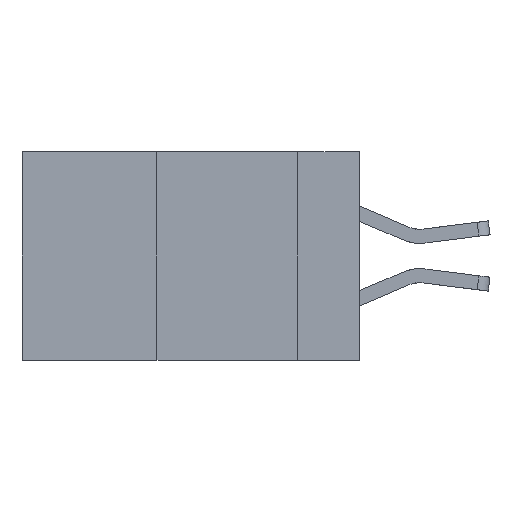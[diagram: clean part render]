
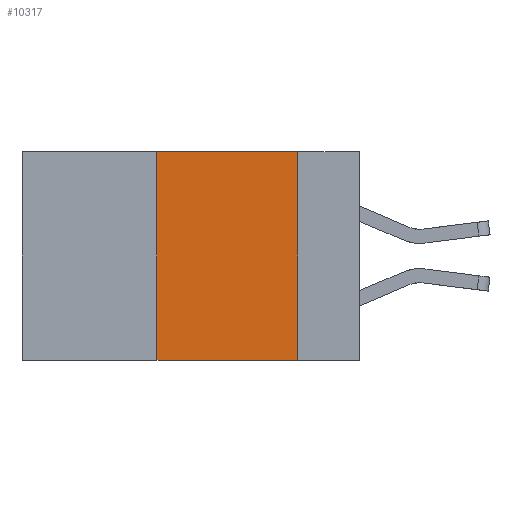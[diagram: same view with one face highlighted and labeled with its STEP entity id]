
A CAD part, left-side view. The second image highlights one B-rep face of the part: STEP entity #10317.
In plain terms, the highlighted planar face has unit normal (-1, 0, 0).
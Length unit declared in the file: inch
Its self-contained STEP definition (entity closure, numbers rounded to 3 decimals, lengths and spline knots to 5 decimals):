
#854 = VECTOR ( 'NONE', #16320, 39.37008 ) ;
#1906 = VECTOR ( 'NONE', #15394, 39.37008 ) ;
#2487 = LINE ( 'NONE', #2749, #8950 ) ;
#2667 = ORIENTED_EDGE ( 'NONE', *, *, #12969, .F. ) ;
#2749 = CARTESIAN_POINT ( 'NONE',  ( 0., 0.6, -0.37 ) ) ;
#3120 = DIRECTION ( 'NONE',  ( 0., 0., -1. ) ) ;
#3386 = VERTEX_POINT ( 'NONE', #4968 ) ;
#3790 = VERTEX_POINT ( 'NONE', #15753 ) ;
#4628 = EDGE_CURVE ( 'NONE', #3386, #15463, #11098, .T. ) ;
#4667 = ORIENTED_EDGE ( 'NONE', *, *, #4628, .F. ) ;
#4968 = CARTESIAN_POINT ( 'NONE',  ( 0., 0.11, 0. ) ) ;
#5385 = DIRECTION ( 'NONE',  ( 0., -1., 0. ) ) ;
#5990 = FACE_OUTER_BOUND ( 'NONE', #14815, .T. ) ;
#7098 = DIRECTION ( 'NONE',  ( 0., -1., 0. ) ) ;
#7210 = LINE ( 'NONE', #14606, #13504 ) ;
#8582 = EDGE_CURVE ( 'NONE', #10566, #3386, #7210, .T. ) ;
#8765 = LINE ( 'NONE', #13083, #1906 ) ;
#8950 = VECTOR ( 'NONE', #5385, 39.37008 ) ;
#9556 = PLANE ( 'NONE',  #10444 ) ;
#9952 = CARTESIAN_POINT ( 'NONE',  ( 0., 0.11, -0.37 ) ) ;
#10317 = ADVANCED_FACE ( 'NONE', ( #5990 ), #9556, .F. ) ;
#10444 = AXIS2_PLACEMENT_3D ( 'NONE', #11962, #10778, #3120 ) ;
#10566 = VERTEX_POINT ( 'NONE', #16106 ) ;
#10778 = DIRECTION ( 'NONE',  ( 1., 0., 0. ) ) ;
#11098 = LINE ( 'NONE', #11379, #854 ) ;
#11379 = CARTESIAN_POINT ( 'NONE',  ( 0., 0.11, 0. ) ) ;
#11962 = CARTESIAN_POINT ( 'NONE',  ( 0., 0.6, 0. ) ) ;
#12969 = EDGE_CURVE ( 'NONE', #3790, #10566, #8765, .T. ) ;
#13083 = CARTESIAN_POINT ( 'NONE',  ( 0., 0.36, 0. ) ) ;
#13504 = VECTOR ( 'NONE', #7098, 39.37008 ) ;
#13596 = EDGE_CURVE ( 'NONE', #3790, #15463, #2487, .T. ) ;
#14347 = ORIENTED_EDGE ( 'NONE', *, *, #8582, .F. ) ;
#14606 = CARTESIAN_POINT ( 'NONE',  ( 0., 0.6, 0. ) ) ;
#14815 = EDGE_LOOP ( 'NONE', ( #4667, #14347, #2667, #16159 ) ) ;
#15394 = DIRECTION ( 'NONE',  ( 0., 0., 1. ) ) ;
#15463 = VERTEX_POINT ( 'NONE', #9952 ) ;
#15753 = CARTESIAN_POINT ( 'NONE',  ( 0., 0.36, -0.37 ) ) ;
#16106 = CARTESIAN_POINT ( 'NONE',  ( 0., 0.36, 0. ) ) ;
#16159 = ORIENTED_EDGE ( 'NONE', *, *, #13596, .T. ) ;
#16320 = DIRECTION ( 'NONE',  ( 0., 0., -1. ) ) ;
